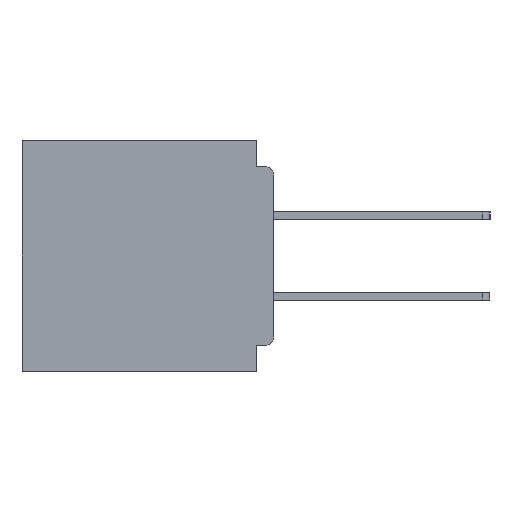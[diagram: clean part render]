
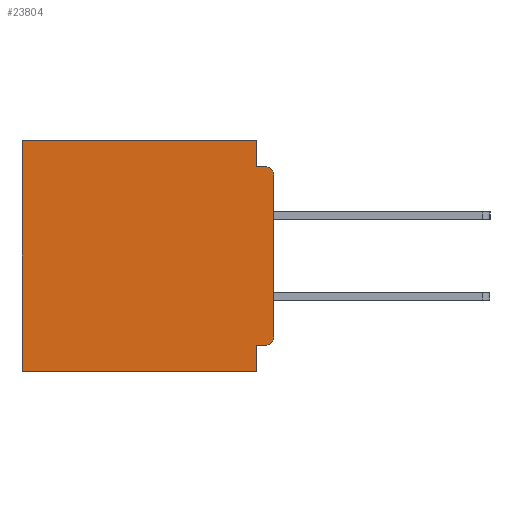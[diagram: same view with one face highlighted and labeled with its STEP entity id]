
A CAD part, left-side view. The second image highlights one B-rep face of the part: STEP entity #23804.
In plain terms, the highlighted planar face has unit normal (-1, 0, 0).
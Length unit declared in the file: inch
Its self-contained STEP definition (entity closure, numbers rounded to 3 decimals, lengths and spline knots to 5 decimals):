
#1156 = VECTOR ( 'NONE', #42641, 39.37008 ) ;
#2237 = EDGE_CURVE ( 'NONE', #36720, #24114, #47197, .T. ) ;
#2563 = ORIENTED_EDGE ( 'NONE', *, *, #29334, .F. ) ;
#2740 = DIRECTION ( 'NONE',  ( 0., 1., 0. ) ) ;
#4075 = VERTEX_POINT ( 'NONE', #40739 ) ;
#4295 = AXIS2_PLACEMENT_3D ( 'NONE', #38718, #25128, #57046 ) ;
#4980 = EDGE_CURVE ( 'NONE', #24114, #49347, #41936, .T. ) ;
#5041 = LINE ( 'NONE', #14970, #29403 ) ;
#5667 = CARTESIAN_POINT ( 'NONE',  ( 0.3, 0.015, -0.045 ) ) ;
#7155 = VECTOR ( 'NONE', #44423, 39.37008 ) ;
#8008 = ORIENTED_EDGE ( 'NONE', *, *, #10553, .T. ) ;
#8591 = LINE ( 'NONE', #16994, #7155 ) ;
#9078 = DIRECTION ( 'NONE',  ( -1., 0., 0. ) ) ;
#9236 = EDGE_CURVE ( 'NONE', #50628, #57916, #8591, .T. ) ;
#9281 = VECTOR ( 'NONE', #47779, 39.37008 ) ;
#10553 = EDGE_CURVE ( 'NONE', #50628, #4075, #54186, .T. ) ;
#11417 = VECTOR ( 'NONE', #18951, 39.37008 ) ;
#13193 = LINE ( 'NONE', #45959, #48288 ) ;
#14332 = CARTESIAN_POINT ( 'NONE',  ( 0.3, 0., -0.045 ) ) ;
#14970 = CARTESIAN_POINT ( 'NONE',  ( 0.3, 0., -0.4 ) ) ;
#15203 = CARTESIAN_POINT ( 'NONE',  ( 0.3, 0.437, -0.4 ) ) ;
#16864 = VECTOR ( 'NONE', #2740, 39.37008 ) ;
#16994 = CARTESIAN_POINT ( 'NONE',  ( 0.3, 0., -0.355 ) ) ;
#17343 = EDGE_CURVE ( 'NONE', #37013, #57758, #46478, .T. ) ;
#17870 = CARTESIAN_POINT ( 'NONE',  ( 0.3, 0.437, 0. ) ) ;
#18218 = CARTESIAN_POINT ( 'NONE',  ( 0.3, 0., -0.06 ) ) ;
#18700 = EDGE_CURVE ( 'NONE', #27119, #4075, #5041, .T. ) ;
#18951 = DIRECTION ( 'NONE',  ( 0., -1., 0. ) ) ;
#19595 = VECTOR ( 'NONE', #54928, 39.37008 ) ;
#20012 = ORIENTED_EDGE ( 'NONE', *, *, #21670, .F. ) ;
#21334 = CIRCLE ( 'NONE', #41237, 0.015 ) ;
#21670 = EDGE_CURVE ( 'NONE', #36720, #37013, #13193, .T. ) ;
#22113 = CARTESIAN_POINT ( 'NONE',  ( 0.3, 0.437, -0.4 ) ) ;
#22761 = CARTESIAN_POINT ( 'NONE',  ( 0.3, 0.015, -0.355 ) ) ;
#23160 = DIRECTION ( 'NONE',  ( 0., 0., -1. ) ) ;
#23804 = ADVANCED_FACE ( 'NONE', ( #49696 ), #52492, .F. ) ;
#24114 = VERTEX_POINT ( 'NONE', #17870 ) ;
#25128 = DIRECTION ( 'NONE',  ( 1., 0., 0. ) ) ;
#27119 = VERTEX_POINT ( 'NONE', #18218 ) ;
#27122 = CARTESIAN_POINT ( 'NONE',  ( 0.3, 0.015, -0.06 ) ) ;
#29334 = EDGE_CURVE ( 'NONE', #33218, #49347, #53367, .T. ) ;
#29403 = VECTOR ( 'NONE', #47011, 39.37008 ) ;
#30247 = AXIS2_PLACEMENT_3D ( 'NONE', #36497, #9078, #41080 ) ;
#31693 = DIRECTION ( 'NONE',  ( 0., 0., -1. ) ) ;
#33218 = VERTEX_POINT ( 'NONE', #35517 ) ;
#35237 = ORIENTED_EDGE ( 'NONE', *, *, #17343, .F. ) ;
#35517 = CARTESIAN_POINT ( 'NONE',  ( 0.3, 0.031, -0.4 ) ) ;
#36497 = CARTESIAN_POINT ( 'NONE',  ( 0.3, 0.015, -0.34 ) ) ;
#36610 = CARTESIAN_POINT ( 'NONE',  ( 0.3, 0.031, -0.4 ) ) ;
#36720 = VERTEX_POINT ( 'NONE', #44195 ) ;
#37013 = VERTEX_POINT ( 'NONE', #46842 ) ;
#38718 = CARTESIAN_POINT ( 'NONE',  ( 0.3, 0., -0.4 ) ) ;
#40739 = CARTESIAN_POINT ( 'NONE',  ( 0.3, 0., -0.34 ) ) ;
#41080 = DIRECTION ( 'NONE',  ( 0., 0., -1. ) ) ;
#41237 = AXIS2_PLACEMENT_3D ( 'NONE', #27122, #58972, #31693 ) ;
#41936 = LINE ( 'NONE', #15203, #1156 ) ;
#42186 = ORIENTED_EDGE ( 'NONE', *, *, #4980, .T. ) ;
#42641 = DIRECTION ( 'NONE',  ( 0., 0., -1. ) ) ;
#43230 = EDGE_CURVE ( 'NONE', #27119, #57758, #21334, .T. ) ;
#44195 = CARTESIAN_POINT ( 'NONE',  ( 0.3, 0.031, 0. ) ) ;
#44423 = DIRECTION ( 'NONE',  ( 0., 1., 0. ) ) ;
#45959 = CARTESIAN_POINT ( 'NONE',  ( 0.3, 0.031, 0. ) ) ;
#46478 = LINE ( 'NONE', #14332, #11417 ) ;
#46842 = CARTESIAN_POINT ( 'NONE',  ( 0.3, 0.031, -0.045 ) ) ;
#47011 = DIRECTION ( 'NONE',  ( 0., 0., -1. ) ) ;
#47063 = ORIENTED_EDGE ( 'NONE', *, *, #43230, .T. ) ;
#47197 = LINE ( 'NONE', #47902, #9281 ) ;
#47779 = DIRECTION ( 'NONE',  ( 0., 1., 0. ) ) ;
#47902 = CARTESIAN_POINT ( 'NONE',  ( 0.3, 0., 0. ) ) ;
#48288 = VECTOR ( 'NONE', #23160, 39.37008 ) ;
#48659 = ORIENTED_EDGE ( 'NONE', *, *, #2237, .T. ) ;
#49347 = VERTEX_POINT ( 'NONE', #22113 ) ;
#49696 = FACE_OUTER_BOUND ( 'NONE', #56258, .T. ) ;
#50628 = VERTEX_POINT ( 'NONE', #22761 ) ;
#50920 = ORIENTED_EDGE ( 'NONE', *, *, #18700, .F. ) ;
#52407 = ORIENTED_EDGE ( 'NONE', *, *, #9236, .F. ) ;
#52492 = PLANE ( 'NONE',  #4295 ) ;
#53367 = LINE ( 'NONE', #57437, #16864 ) ;
#54186 = CIRCLE ( 'NONE', #30247, 0.015 ) ;
#54928 = DIRECTION ( 'NONE',  ( 0., 0., -1. ) ) ;
#55087 = EDGE_CURVE ( 'NONE', #57916, #33218, #57482, .T. ) ;
#56258 = EDGE_LOOP ( 'NONE', ( #50920, #47063, #35237, #20012, #48659, #42186, #2563, #57453, #52407, #8008 ) ) ;
#56969 = CARTESIAN_POINT ( 'NONE',  ( 0.3, 0.031, -0.355 ) ) ;
#57046 = DIRECTION ( 'NONE',  ( 0., 0., -1. ) ) ;
#57437 = CARTESIAN_POINT ( 'NONE',  ( 0.3, 0., -0.4 ) ) ;
#57453 = ORIENTED_EDGE ( 'NONE', *, *, #55087, .F. ) ;
#57482 = LINE ( 'NONE', #36610, #19595 ) ;
#57758 = VERTEX_POINT ( 'NONE', #5667 ) ;
#57916 = VERTEX_POINT ( 'NONE', #56969 ) ;
#58972 = DIRECTION ( 'NONE',  ( -1., 0., 0. ) ) ;
